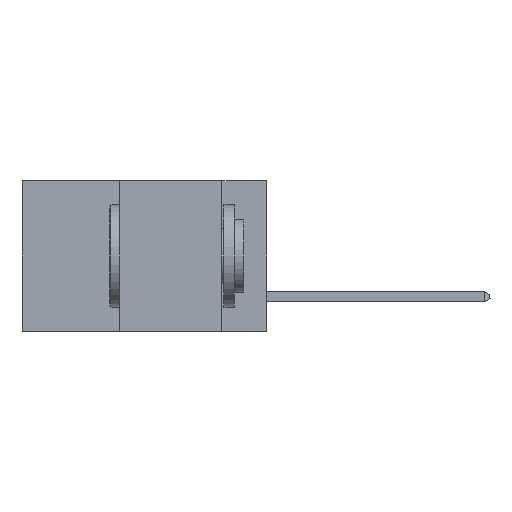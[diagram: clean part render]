
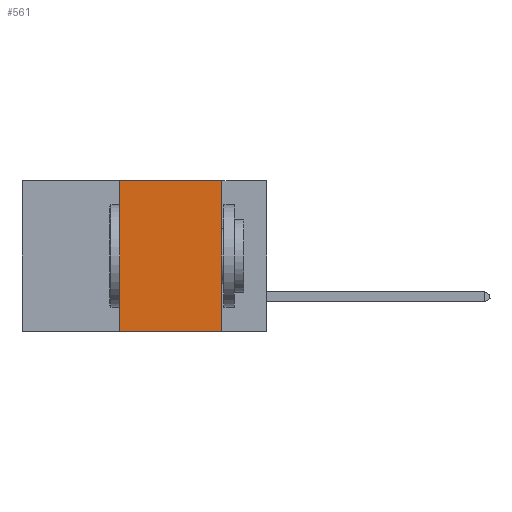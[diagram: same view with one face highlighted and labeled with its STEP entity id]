
A CAD part, left-side view. The second image highlights one B-rep face of the part: STEP entity #561.
In plain terms, the highlighted planar face has unit normal (-1, 0, 0).
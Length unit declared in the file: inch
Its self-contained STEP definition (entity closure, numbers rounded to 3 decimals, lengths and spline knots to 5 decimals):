
#471 = EDGE_CURVE ( 'NONE', #4606, #2203, #7683, .T. ) ;
#561 = ADVANCED_FACE ( 'NONE', ( #12993 ), #10026, .F. ) ;
#618 = VERTEX_POINT ( 'NONE', #1094 ) ;
#674 = DIRECTION ( 'NONE',  ( 0., 0., -1. ) ) ;
#700 = CARTESIAN_POINT ( 'NONE',  ( 0., 0.36, 0. ) ) ;
#1094 = CARTESIAN_POINT ( 'NONE',  ( 0., 0.11, -0.37 ) ) ;
#2203 = VERTEX_POINT ( 'NONE', #15295 ) ;
#3199 = EDGE_CURVE ( 'NONE', #10234, #618, #22913, .T. ) ;
#3406 = EDGE_CURVE ( 'NONE', #2203, #618, #19106, .T. ) ;
#3688 = LINE ( 'NONE', #6316, #12295 ) ;
#4606 = VERTEX_POINT ( 'NONE', #700 ) ;
#5457 = DIRECTION ( 'NONE',  ( 0., 0., -1. ) ) ;
#5502 = CARTESIAN_POINT ( 'NONE',  ( 0., 0.6, 0. ) ) ;
#6211 = DIRECTION ( 'NONE',  ( 0., 0., 1. ) ) ;
#6316 = CARTESIAN_POINT ( 'NONE',  ( 0., 0.36, 0. ) ) ;
#7683 = LINE ( 'NONE', #8164, #15239 ) ;
#7941 = DIRECTION ( 'NONE',  ( 0., -1., 0. ) ) ;
#8164 = CARTESIAN_POINT ( 'NONE',  ( 0., 0.6, 0. ) ) ;
#10026 = PLANE ( 'NONE',  #27608 ) ;
#10234 = VERTEX_POINT ( 'NONE', #17886 ) ;
#11893 = ORIENTED_EDGE ( 'NONE', *, *, #3406, .F. ) ;
#12295 = VECTOR ( 'NONE', #6211, 39.37008 ) ;
#12993 = FACE_OUTER_BOUND ( 'NONE', #25409, .T. ) ;
#15239 = VECTOR ( 'NONE', #7941, 39.37008 ) ;
#15295 = CARTESIAN_POINT ( 'NONE',  ( 0., 0.11, 0. ) ) ;
#16019 = ORIENTED_EDGE ( 'NONE', *, *, #3199, .T. ) ;
#17239 = VECTOR ( 'NONE', #5457, 39.37008 ) ;
#17886 = CARTESIAN_POINT ( 'NONE',  ( 0., 0.36, -0.37 ) ) ;
#19106 = LINE ( 'NONE', #22268, #17239 ) ;
#20794 = ORIENTED_EDGE ( 'NONE', *, *, #471, .F. ) ;
#22268 = CARTESIAN_POINT ( 'NONE',  ( 0., 0.11, 0. ) ) ;
#22287 = ORIENTED_EDGE ( 'NONE', *, *, #29988, .F. ) ;
#22913 = LINE ( 'NONE', #30981, #25946 ) ;
#25409 = EDGE_LOOP ( 'NONE', ( #11893, #20794, #22287, #16019 ) ) ;
#25824 = DIRECTION ( 'NONE',  ( 0., -1., 0. ) ) ;
#25946 = VECTOR ( 'NONE', #25824, 39.37008 ) ;
#27188 = DIRECTION ( 'NONE',  ( 1., 0., 0. ) ) ;
#27608 = AXIS2_PLACEMENT_3D ( 'NONE', #5502, #27188, #674 ) ;
#29988 = EDGE_CURVE ( 'NONE', #10234, #4606, #3688, .T. ) ;
#30981 = CARTESIAN_POINT ( 'NONE',  ( 0., 0.6, -0.37 ) ) ;
